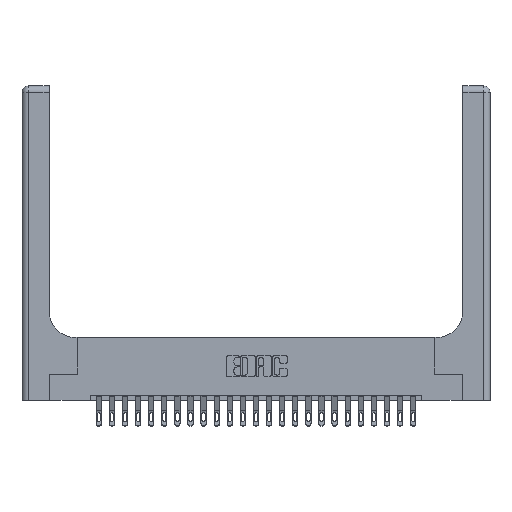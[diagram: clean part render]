
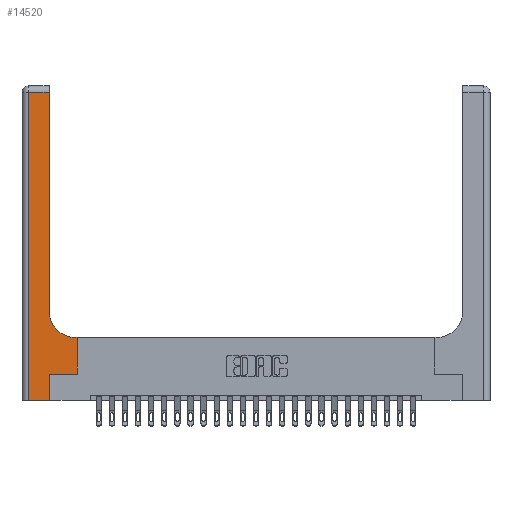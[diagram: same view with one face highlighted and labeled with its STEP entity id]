
A CAD part, top view. The second image highlights one B-rep face of the part: STEP entity #14520.
In plain terms, the highlighted planar face has unit normal (0, 0, 1).
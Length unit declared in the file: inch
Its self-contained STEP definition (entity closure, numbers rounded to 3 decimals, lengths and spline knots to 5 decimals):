
#286 = CARTESIAN_POINT ( 'NONE',  ( 0.265, 0.25, 0.37 ) ) ;
#363 = DIRECTION ( 'NONE',  ( 1., 0., 0. ) ) ;
#510 = DIRECTION ( 'NONE',  ( 0., 0., -1. ) ) ;
#871 = VECTOR ( 'NONE', #3113, 39.37008 ) ;
#1616 = ORIENTED_EDGE ( 'NONE', *, *, #21519, .T. ) ;
#1935 = VERTEX_POINT ( 'NONE', #19527 ) ;
#2074 = AXIS2_PLACEMENT_3D ( 'NONE', #5860, #22853, #13201 ) ;
#2139 = CARTESIAN_POINT ( 'NONE',  ( 0.26, 0.85, 0.37 ) ) ;
#3050 = VERTEX_POINT ( 'NONE', #13329 ) ;
#3113 = DIRECTION ( 'NONE',  ( 1., 0., 0. ) ) ;
#3214 = FACE_OUTER_BOUND ( 'NONE', #3920, .T. ) ;
#3804 = DIRECTION ( 'NONE',  ( -1., 0., 0. ) ) ;
#3920 = EDGE_LOOP ( 'NONE', ( #5141, #23210, #20876, #22412, #19892, #20119, #1616, #6066, #16933 ) ) ;
#3984 = AXIS2_PLACEMENT_3D ( 'NONE', #8035, #510, #10056 ) ;
#4004 = DIRECTION ( 'NONE',  ( 0., -1., 0. ) ) ;
#4376 = VECTOR ( 'NONE', #363, 39.37008 ) ;
#4660 = CARTESIAN_POINT ( 'NONE',  ( 0.265, 0., 0.37 ) ) ;
#4828 = EDGE_CURVE ( 'NONE', #23560, #7351, #11257, .T. ) ;
#5087 = VECTOR ( 'NONE', #4004, 39.37008 ) ;
#5141 = ORIENTED_EDGE ( 'NONE', *, *, #11662, .T. ) ;
#5860 = CARTESIAN_POINT ( 'NONE',  ( 0.51, 0.85, 0.37 ) ) ;
#6066 = ORIENTED_EDGE ( 'NONE', *, *, #17233, .T. ) ;
#6744 = CARTESIAN_POINT ( 'NONE',  ( 0., 0., 0.37 ) ) ;
#6992 = CARTESIAN_POINT ( 'NONE',  ( 0., 2.94, 0.37 ) ) ;
#7351 = VERTEX_POINT ( 'NONE', #4660 ) ;
#7934 = PLANE ( 'NONE',  #3984 ) ;
#8035 = CARTESIAN_POINT ( 'NONE',  ( 0., 3., 0.37 ) ) ;
#8986 = LINE ( 'NONE', #286, #4376 ) ;
#9080 = EDGE_CURVE ( 'NONE', #10628, #23560, #15883, .T. ) ;
#9146 = CARTESIAN_POINT ( 'NONE',  ( 0.06, 2.94, 0.37 ) ) ;
#9282 = VECTOR ( 'NONE', #19839, 39.37008 ) ;
#9310 = CARTESIAN_POINT ( 'NONE',  ( 0.26, 0.6, 0.37 ) ) ;
#9384 = EDGE_CURVE ( 'NONE', #7351, #1935, #16458, .T. ) ;
#9485 = CARTESIAN_POINT ( 'NONE',  ( 0.528, 0.25, 0.37 ) ) ;
#9749 = VERTEX_POINT ( 'NONE', #9485 ) ;
#10056 = DIRECTION ( 'NONE',  ( -1., 0., 0. ) ) ;
#10628 = VERTEX_POINT ( 'NONE', #9146 ) ;
#11257 = LINE ( 'NONE', #6744, #871 ) ;
#11607 = VECTOR ( 'NONE', #21032, 39.37008 ) ;
#11662 = EDGE_CURVE ( 'NONE', #18562, #3050, #22519, .T. ) ;
#12072 = LINE ( 'NONE', #9310, #23558 ) ;
#12161 = EDGE_CURVE ( 'NONE', #3050, #10628, #18363, .T. ) ;
#13201 = DIRECTION ( 'NONE',  ( 1., 0., 0. ) ) ;
#13329 = CARTESIAN_POINT ( 'NONE',  ( 0.26, 2.94, 0.37 ) ) ;
#14491 = EDGE_CURVE ( 'NONE', #1935, #9749, #8986, .T. ) ;
#14520 = ADVANCED_FACE ( 'NONE', ( #3214 ), #7934, .F. ) ;
#14796 = CARTESIAN_POINT ( 'NONE',  ( 0.51, 0.6, 0.37 ) ) ;
#15211 = DIRECTION ( 'NONE',  ( 0., 1., 0. ) ) ;
#15883 = LINE ( 'NONE', #18519, #5087 ) ;
#16458 = LINE ( 'NONE', #18976, #23216 ) ;
#16933 = ORIENTED_EDGE ( 'NONE', *, *, #20024, .T. ) ;
#17233 = EDGE_CURVE ( 'NONE', #19826, #17442, #12072, .T. ) ;
#17442 = VERTEX_POINT ( 'NONE', #14796 ) ;
#17503 = CARTESIAN_POINT ( 'NONE',  ( 0.26, 3., 0.37 ) ) ;
#18148 = LINE ( 'NONE', #20198, #21969 ) ;
#18363 = LINE ( 'NONE', #6992, #9282 ) ;
#18440 = DIRECTION ( 'NONE',  ( 0., 1., 0. ) ) ;
#18519 = CARTESIAN_POINT ( 'NONE',  ( 0.06, 3., 0.37 ) ) ;
#18562 = VERTEX_POINT ( 'NONE', #2139 ) ;
#18976 = CARTESIAN_POINT ( 'NONE',  ( 0.265, 0., 0.37 ) ) ;
#19527 = CARTESIAN_POINT ( 'NONE',  ( 0.265, 0.25, 0.37 ) ) ;
#19826 = VERTEX_POINT ( 'NONE', #20200 ) ;
#19839 = DIRECTION ( 'NONE',  ( -1., 0., 0. ) ) ;
#19892 = ORIENTED_EDGE ( 'NONE', *, *, #9384, .T. ) ;
#20024 = EDGE_CURVE ( 'NONE', #17442, #18562, #24024, .T. ) ;
#20119 = ORIENTED_EDGE ( 'NONE', *, *, #14491, .T. ) ;
#20198 = CARTESIAN_POINT ( 'NONE',  ( 0.528, 0.25, 0.37 ) ) ;
#20200 = CARTESIAN_POINT ( 'NONE',  ( 0.528, 0.6, 0.37 ) ) ;
#20336 = CARTESIAN_POINT ( 'NONE',  ( 0.06, 0., 0.37 ) ) ;
#20876 = ORIENTED_EDGE ( 'NONE', *, *, #9080, .T. ) ;
#21032 = DIRECTION ( 'NONE',  ( 0., 1., 0. ) ) ;
#21519 = EDGE_CURVE ( 'NONE', #9749, #19826, #18148, .T. ) ;
#21969 = VECTOR ( 'NONE', #18440, 39.37008 ) ;
#22412 = ORIENTED_EDGE ( 'NONE', *, *, #4828, .T. ) ;
#22519 = LINE ( 'NONE', #17503, #11607 ) ;
#22853 = DIRECTION ( 'NONE',  ( 0., 0., -1. ) ) ;
#23210 = ORIENTED_EDGE ( 'NONE', *, *, #12161, .T. ) ;
#23216 = VECTOR ( 'NONE', #15211, 39.37008 ) ;
#23558 = VECTOR ( 'NONE', #3804, 39.37008 ) ;
#23560 = VERTEX_POINT ( 'NONE', #20336 ) ;
#24024 = CIRCLE ( 'NONE', #2074, 0.25 ) ;
